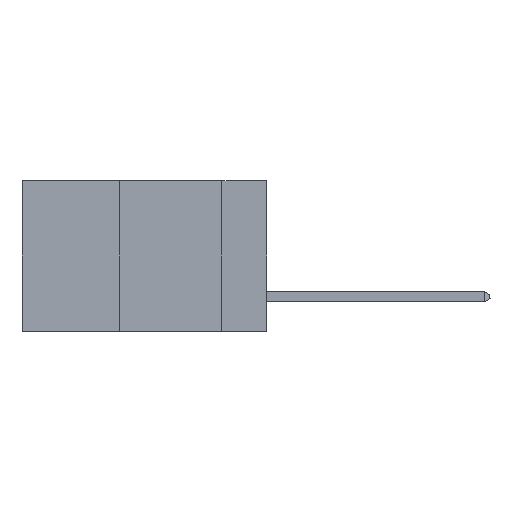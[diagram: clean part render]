
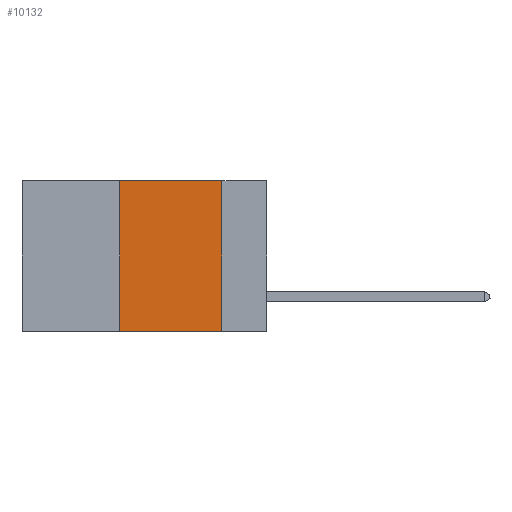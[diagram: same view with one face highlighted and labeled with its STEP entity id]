
A CAD part, left-side view. The second image highlights one B-rep face of the part: STEP entity #10132.
In plain terms, the highlighted planar face has unit normal (-1, 0, 0).
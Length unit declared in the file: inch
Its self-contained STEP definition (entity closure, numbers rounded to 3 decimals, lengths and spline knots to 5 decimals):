
#344 = PLANE ( 'NONE',  #6466 ) ;
#1061 = ORIENTED_EDGE ( 'NONE', *, *, #12230, .F. ) ;
#1972 = CARTESIAN_POINT ( 'NONE',  ( 0., 0.11, 0. ) ) ;
#2622 = EDGE_CURVE ( 'NONE', #5375, #8738, #3306, .T. ) ;
#2957 = EDGE_CURVE ( 'NONE', #5375, #7641, #5208, .T. ) ;
#3150 = VECTOR ( 'NONE', #3335, 39.37008 ) ;
#3306 = LINE ( 'NONE', #3377, #3150 ) ;
#3335 = DIRECTION ( 'NONE',  ( 0., -1., 0. ) ) ;
#3377 = CARTESIAN_POINT ( 'NONE',  ( 0., 0.6, -0.37 ) ) ;
#3425 = CARTESIAN_POINT ( 'NONE',  ( 0., 0.36, -0.37 ) ) ;
#3528 = ORIENTED_EDGE ( 'NONE', *, *, #2622, .T. ) ;
#3822 = LINE ( 'NONE', #8176, #8141 ) ;
#4904 = EDGE_CURVE ( 'NONE', #9773, #8738, #11810, .T. ) ;
#5208 = LINE ( 'NONE', #7088, #8883 ) ;
#5375 = VERTEX_POINT ( 'NONE', #3425 ) ;
#5938 = CARTESIAN_POINT ( 'NONE',  ( 0., 0.36, 0. ) ) ;
#5988 = EDGE_LOOP ( 'NONE', ( #8415, #1061, #7463, #3528 ) ) ;
#6466 = AXIS2_PLACEMENT_3D ( 'NONE', #11498, #12491, #7642 ) ;
#6899 = FACE_OUTER_BOUND ( 'NONE', #5988, .T. ) ;
#7088 = CARTESIAN_POINT ( 'NONE',  ( 0., 0.36, 0. ) ) ;
#7463 = ORIENTED_EDGE ( 'NONE', *, *, #2957, .F. ) ;
#7641 = VERTEX_POINT ( 'NONE', #5938 ) ;
#7642 = DIRECTION ( 'NONE',  ( 0., 0., -1. ) ) ;
#7891 = DIRECTION ( 'NONE',  ( 0., 0., -1. ) ) ;
#8141 = VECTOR ( 'NONE', #11238, 39.37008 ) ;
#8176 = CARTESIAN_POINT ( 'NONE',  ( 0., 0.6, 0. ) ) ;
#8415 = ORIENTED_EDGE ( 'NONE', *, *, #4904, .F. ) ;
#8738 = VERTEX_POINT ( 'NONE', #9604 ) ;
#8883 = VECTOR ( 'NONE', #11039, 39.37008 ) ;
#9604 = CARTESIAN_POINT ( 'NONE',  ( 0., 0.11, -0.37 ) ) ;
#9773 = VERTEX_POINT ( 'NONE', #1972 ) ;
#10132 = ADVANCED_FACE ( 'NONE', ( #6899 ), #344, .F. ) ;
#11039 = DIRECTION ( 'NONE',  ( 0., 0., 1. ) ) ;
#11238 = DIRECTION ( 'NONE',  ( 0., -1., 0. ) ) ;
#11498 = CARTESIAN_POINT ( 'NONE',  ( 0., 0.6, 0. ) ) ;
#11810 = LINE ( 'NONE', #11910, #12767 ) ;
#11910 = CARTESIAN_POINT ( 'NONE',  ( 0., 0.11, 0. ) ) ;
#12230 = EDGE_CURVE ( 'NONE', #7641, #9773, #3822, .T. ) ;
#12491 = DIRECTION ( 'NONE',  ( 1., 0., 0. ) ) ;
#12767 = VECTOR ( 'NONE', #7891, 39.37008 ) ;
